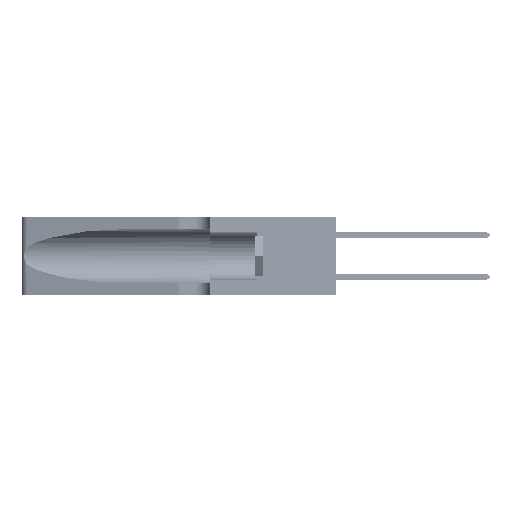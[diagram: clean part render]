
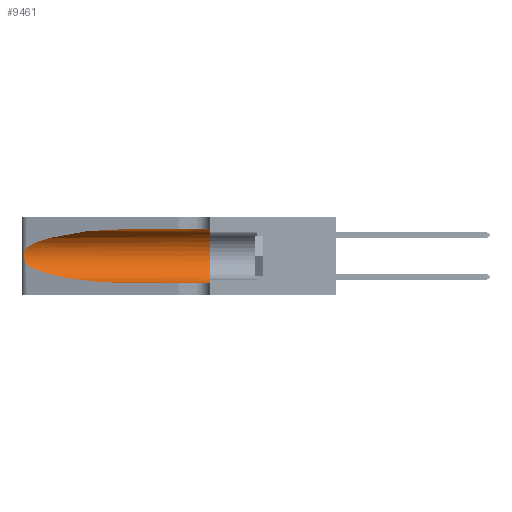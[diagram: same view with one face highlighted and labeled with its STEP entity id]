
A CAD part, left-side view. The second image highlights one B-rep face of the part: STEP entity #9461.
In plain terms, the highlighted cylindrical face has radius 3.308 mm (diameter 6.617 mm), a partial arc.
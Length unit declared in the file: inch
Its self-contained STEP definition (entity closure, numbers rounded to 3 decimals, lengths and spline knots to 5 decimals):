
#21 = EDGE_CURVE ( 'NONE', #31104, #31659, #8973, .T. ) ;
#1446 = CYLINDRICAL_SURFACE ( 'NONE', #35212, 0.13025 ) ;
#1970 = CARTESIAN_POINT ( 'NONE',  ( 0.25487, 1.22718, 0.14631 ) ) ;
#4373 = CARTESIAN_POINT ( 'NONE',  ( 0.2373, 1.15595, 0.28018 ) ) ;
#5692 =( BOUNDED_CURVE ( )  B_SPLINE_CURVE ( 3, ( #1970, #10183, #30525, #46865 ),
 .UNSPECIFIED., .F., .F. ) 
 B_SPLINE_CURVE_WITH_KNOTS ( ( 4, 4 ),
 ( 3.44316, 4.71239 ),
 .UNSPECIFIED. ) 
 CURVE ( )  GEOMETRIC_REPRESENTATION_ITEM ( )  RATIONAL_B_SPLINE_CURVE ( ( 1., 0.87, 0.87, 1. ) ) 
 REPRESENTATION_ITEM ( '' )  );
#7040 = CARTESIAN_POINT ( 'NONE',  ( 0.25487, 1.22718, 0.22369 ) ) ;
#7510 = DIRECTION ( 'NONE',  ( 0., -1., 0. ) ) ;
#8973 = LINE ( 'NONE', #44697, #28064 ) ;
#9461 = ADVANCED_FACE ( 'NONE', ( #25700 ), #1446, .F. ) ;
#9770 = EDGE_CURVE ( 'NONE', #31659, #25725, #17362, .T. ) ;
#10183 = CARTESIAN_POINT ( 'NONE',  ( 0.2373, 1.15595, 0.08982 ) ) ;
#10585 = VECTOR ( 'NONE', #45994, 39.37008 ) ;
#10602 = VERTEX_POINT ( 'NONE', #7040 ) ;
#10873 = CARTESIAN_POINT ( 'NONE',  ( 0.26017, 1.23833, 0.17102 ) ) ;
#11224 = CARTESIAN_POINT ( 'NONE',  ( 0.25854, 1.2359, 0.20912 ) ) ;
#11611 = ORIENTED_EDGE ( 'NONE', *, *, #23756, .T. ) ;
#11950 = CARTESIAN_POINT ( 'NONE',  ( 0.1305, 1.61858, 0.185 ) ) ;
#12125 = ORIENTED_EDGE ( 'NONE', *, *, #9770, .F. ) ;
#12942 = CARTESIAN_POINT ( 'NONE',  ( 0.25487, 1.22718, 0.22369 ) ) ;
#13361 = AXIS2_PLACEMENT_3D ( 'NONE', #30589, #14022, #46569 ) ;
#14022 = DIRECTION ( 'NONE',  ( 0., 1., 0. ) ) ;
#15681 = CARTESIAN_POINT ( 'NONE',  ( 0.25639, 1.23186, 0.15144 ) ) ;
#15698 = DIRECTION ( 'NONE',  ( 0., 0., -1. ) ) ;
#15723 = CARTESIAN_POINT ( 'NONE',  ( 0.1305, 0.72297, 0.31525 ) ) ;
#17244 = ORIENTED_EDGE ( 'NONE', *, *, #46886, .T. ) ;
#17362 = CIRCLE ( 'NONE', #13361, 0.13025 ) ;
#19441 = CARTESIAN_POINT ( 'NONE',  ( 0.26075, 1.23896, 0.19203 ) ) ;
#19617 = CARTESIAN_POINT ( 'NONE',  ( 0.25856, 1.23593, 0.16098 ) ) ;
#20249 = EDGE_CURVE ( 'NONE', #10602, #22587, #46159, .T. ) ;
#20974 = CARTESIAN_POINT ( 'NONE',  ( 0.1305, 0.72297, 0.31525 ) ) ;
#21799 = CARTESIAN_POINT ( 'NONE',  ( 0.1305, 1.61858, 0.05475 ) ) ;
#22587 = VERTEX_POINT ( 'NONE', #38239 ) ;
#23359 = CARTESIAN_POINT ( 'NONE',  ( 0.25639, 1.23184, 0.21858 ) ) ;
#23694 = CARTESIAN_POINT ( 'NONE',  ( 0.25789, 1.23486, 0.15765 ) ) ;
#23756 = EDGE_CURVE ( 'NONE', #31104, #10602, #25613, .T. ) ;
#23881 = EDGE_LOOP ( 'NONE', ( #11611, #33644, #17244, #43116, #12125, #31929 ) ) ;
#24078 = VERTEX_POINT ( 'NONE', #30916 ) ;
#25613 =( BOUNDED_CURVE ( )  B_SPLINE_CURVE ( 3, ( #20974, #33064, #4373, #12942 ),
 .UNSPECIFIED., .F., .F. ) 
 B_SPLINE_CURVE_WITH_KNOTS ( ( 4, 4 ),
 ( 1.5708, 2.84003 ),
 .UNSPECIFIED. ) 
 CURVE ( )  GEOMETRIC_REPRESENTATION_ITEM ( )  RATIONAL_B_SPLINE_CURVE ( ( 1., 0.87, 0.87, 1. ) ) 
 REPRESENTATION_ITEM ( '' )  );
#25700 = FACE_OUTER_BOUND ( 'NONE', #23881, .T. ) ;
#25725 = VERTEX_POINT ( 'NONE', #30184 ) ;
#27428 = CARTESIAN_POINT ( 'NONE',  ( 0.25555, 1.22994, 0.2215 ) ) ;
#27938 = CARTESIAN_POINT ( 'NONE',  ( 0.25487, 1.22718, 0.14631 ) ) ;
#28064 = VECTOR ( 'NONE', #7510, 39.37008 ) ;
#30184 = CARTESIAN_POINT ( 'NONE',  ( 0.1305, 0.35, 0.05475 ) ) ;
#30405 = LINE ( 'NONE', #21799, #10585 ) ;
#30525 = CARTESIAN_POINT ( 'NONE',  ( 0.18966, 0.96281, 0.05475 ) ) ;
#30589 = CARTESIAN_POINT ( 'NONE',  ( 0.1305, 0.35, 0.185 ) ) ;
#30916 = CARTESIAN_POINT ( 'NONE',  ( 0.1305, 0.72297, 0.05475 ) ) ;
#31104 = VERTEX_POINT ( 'NONE', #15723 ) ;
#31659 = VERTEX_POINT ( 'NONE', #40932 ) ;
#31929 = ORIENTED_EDGE ( 'NONE', *, *, #21, .F. ) ;
#33064 = CARTESIAN_POINT ( 'NONE',  ( 0.18966, 0.96281, 0.31525 ) ) ;
#33644 = ORIENTED_EDGE ( 'NONE', *, *, #20249, .T. ) ;
#35212 = AXIS2_PLACEMENT_3D ( 'NONE', #11950, #36179, #15698 ) ;
#36179 = DIRECTION ( 'NONE',  ( 0., -1., 0. ) ) ;
#38239 = CARTESIAN_POINT ( 'NONE',  ( 0.25487, 1.22718, 0.14631 ) ) ;
#39520 = CARTESIAN_POINT ( 'NONE',  ( 0.25487, 1.22718, 0.22369 ) ) ;
#39696 = CARTESIAN_POINT ( 'NONE',  ( 0.26018, 1.23835, 0.19895 ) ) ;
#39878 = CARTESIAN_POINT ( 'NONE',  ( 0.25787, 1.23484, 0.2124 ) ) ;
#40932 = CARTESIAN_POINT ( 'NONE',  ( 0.1305, 0.35, 0.31525 ) ) ;
#41350 = EDGE_CURVE ( 'NONE', #24078, #25725, #30405, .T. ) ;
#43116 = ORIENTED_EDGE ( 'NONE', *, *, #41350, .T. ) ;
#43975 = CARTESIAN_POINT ( 'NONE',  ( 0.26075, 1.23896, 0.178 ) ) ;
#44157 = CARTESIAN_POINT ( 'NONE',  ( 0.25555, 1.22993, 0.14849 ) ) ;
#44697 = CARTESIAN_POINT ( 'NONE',  ( 0.1305, 1.61858, 0.31525 ) ) ;
#45994 = DIRECTION ( 'NONE',  ( 0., -1., 0. ) ) ;
#46159 = B_SPLINE_CURVE_WITH_KNOTS ( 'NONE', 3,
 ( #39520, #27428, #23359, #39878, #11224, #39696, #19441, #43975, #10873, #19617, #23694, #15681, #44157, #27938 ),
 .UNSPECIFIED., .F., .F.,
 ( 4, 2, 2, 2, 2, 2, 4 ),
 ( 0., 0.00027, 0.00053, 0.00107, 0.0016, 0.00187, 0.00214 ),
 .UNSPECIFIED. ) ;
#46569 = DIRECTION ( 'NONE',  ( 0., 0., 1. ) ) ;
#46865 = CARTESIAN_POINT ( 'NONE',  ( 0.1305, 0.72297, 0.05475 ) ) ;
#46886 = EDGE_CURVE ( 'NONE', #22587, #24078, #5692, .T. ) ;
